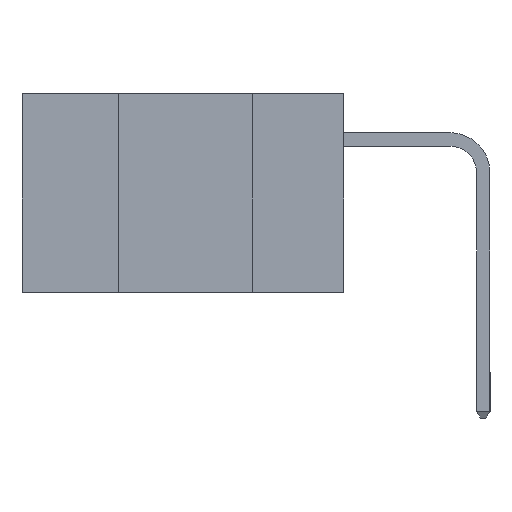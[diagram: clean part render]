
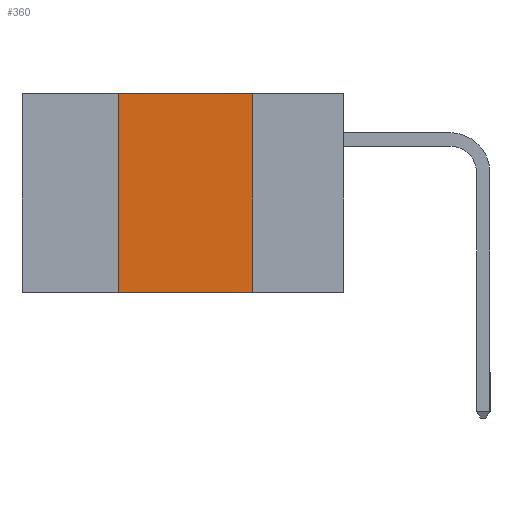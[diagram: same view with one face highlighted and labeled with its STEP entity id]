
A CAD part, left-side view. The second image highlights one B-rep face of the part: STEP entity #360.
In plain terms, the highlighted planar face has unit normal (-1, 0, 0).
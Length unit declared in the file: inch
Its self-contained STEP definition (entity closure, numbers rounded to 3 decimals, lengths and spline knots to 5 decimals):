
#222 = PLANE ( 'NONE',  #8500 ) ;
#360 = ADVANCED_FACE ( 'NONE', ( #3885 ), #222, .F. ) ;
#554 = DIRECTION ( 'NONE',  ( 0., 0., -1. ) ) ;
#579 = CARTESIAN_POINT ( 'NONE',  ( 0., 0.42, -0.37 ) ) ;
#1186 = VECTOR ( 'NONE', #7348, 39.37008 ) ;
#1316 = LINE ( 'NONE', #9208, #2253 ) ;
#1321 = VERTEX_POINT ( 'NONE', #579 ) ;
#1462 = DIRECTION ( 'NONE',  ( 0., 0., 1. ) ) ;
#1545 = ORIENTED_EDGE ( 'NONE', *, *, #12667, .F. ) ;
#2140 = EDGE_LOOP ( 'NONE', ( #1545, #21996, #12162, #20288 ) ) ;
#2253 = VECTOR ( 'NONE', #1462, 39.37008 ) ;
#2397 = VERTEX_POINT ( 'NONE', #17972 ) ;
#3774 = CARTESIAN_POINT ( 'NONE',  ( 0., 0.42, 0. ) ) ;
#3885 = FACE_OUTER_BOUND ( 'NONE', #2140, .T. ) ;
#4391 = CARTESIAN_POINT ( 'NONE',  ( 0., 0.6, 0. ) ) ;
#4819 = LINE ( 'NONE', #8993, #11551 ) ;
#4979 = VERTEX_POINT ( 'NONE', #17759 ) ;
#6906 = EDGE_CURVE ( 'NONE', #15922, #2397, #4819, .T. ) ;
#7348 = DIRECTION ( 'NONE',  ( 0., -1., 0. ) ) ;
#8500 = AXIS2_PLACEMENT_3D ( 'NONE', #4391, #19990, #554 ) ;
#8935 = VECTOR ( 'NONE', #17226, 39.37008 ) ;
#8993 = CARTESIAN_POINT ( 'NONE',  ( 0., 0.6, 0. ) ) ;
#9102 = CARTESIAN_POINT ( 'NONE',  ( 0., 0.17, 0. ) ) ;
#9208 = CARTESIAN_POINT ( 'NONE',  ( 0., 0.42, 0. ) ) ;
#10175 = LINE ( 'NONE', #9102, #8935 ) ;
#11551 = VECTOR ( 'NONE', #22562, 39.37008 ) ;
#12162 = ORIENTED_EDGE ( 'NONE', *, *, #25221, .F. ) ;
#12667 = EDGE_CURVE ( 'NONE', #2397, #4979, #10175, .T. ) ;
#14968 = EDGE_CURVE ( 'NONE', #1321, #4979, #25316, .T. ) ;
#15922 = VERTEX_POINT ( 'NONE', #3774 ) ;
#17226 = DIRECTION ( 'NONE',  ( 0., 0., -1. ) ) ;
#17759 = CARTESIAN_POINT ( 'NONE',  ( 0., 0.17, -0.37 ) ) ;
#17972 = CARTESIAN_POINT ( 'NONE',  ( 0., 0.17, 0. ) ) ;
#19032 = CARTESIAN_POINT ( 'NONE',  ( 0., 0.6, -0.37 ) ) ;
#19990 = DIRECTION ( 'NONE',  ( 1., 0., 0. ) ) ;
#20288 = ORIENTED_EDGE ( 'NONE', *, *, #14968, .T. ) ;
#21996 = ORIENTED_EDGE ( 'NONE', *, *, #6906, .F. ) ;
#22562 = DIRECTION ( 'NONE',  ( 0., -1., 0. ) ) ;
#25221 = EDGE_CURVE ( 'NONE', #1321, #15922, #1316, .T. ) ;
#25316 = LINE ( 'NONE', #19032, #1186 ) ;
